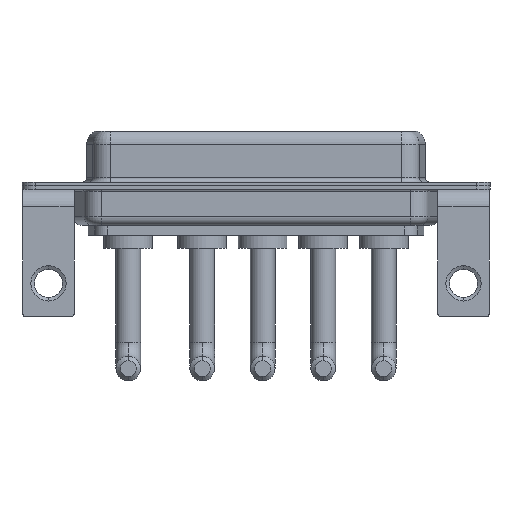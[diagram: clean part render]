
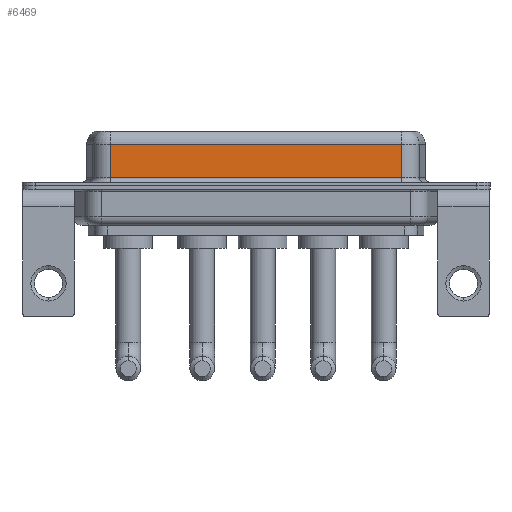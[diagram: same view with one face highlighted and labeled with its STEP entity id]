
A CAD part, front view. The second image highlights one B-rep face of the part: STEP entity #6469.
In plain terms, the highlighted planar face has unit normal (0, -1, 0).
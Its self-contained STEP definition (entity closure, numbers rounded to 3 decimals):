
#188 = CARTESIAN_POINT ( 'NONE',  ( 40.037, -3.95, 0.9 ) ) ;
#1151 = VERTEX_POINT ( 'NONE', #8753 ) ;
#1184 = VERTEX_POINT ( 'NONE', #9587 ) ;
#1342 = DIRECTION ( 'NONE',  ( 1., 0., 0. ) ) ;
#1754 = VECTOR ( 'NONE', #6107, 1000. ) ;
#1805 = VECTOR ( 'NONE', #10194, 1000. ) ;
#2110 = ORIENTED_EDGE ( 'NONE', *, *, #11694, .F. ) ;
#2788 = DIRECTION ( 'NONE',  ( 0., 0., 1. ) ) ;
#2907 = LINE ( 'NONE', #11428, #1754 ) ;
#2915 = LINE ( 'NONE', #6045, #1805 ) ;
#5626 = LINE ( 'NONE', #188, #5764 ) ;
#5632 = VERTEX_POINT ( 'NONE', #7070 ) ;
#5764 = VECTOR ( 'NONE', #1342, 1000. ) ;
#5887 = ORIENTED_EDGE ( 'NONE', *, *, #8038, .T. ) ;
#5916 = FACE_OUTER_BOUND ( 'NONE', #6732, .T. ) ;
#6045 = CARTESIAN_POINT ( 'NONE',  ( 40.037, -3.95, 4.65 ) ) ;
#6107 = DIRECTION ( 'NONE',  ( 0., 0., -1. ) ) ;
#6469 = ADVANCED_FACE ( 'NONE', ( #5916 ), #13076, .F. ) ;
#6732 = EDGE_LOOP ( 'NONE', ( #2110, #5887, #8091, #12828 ) ) ;
#7070 = CARTESIAN_POINT ( 'NONE',  ( 40.037, -3.95, 4.65 ) ) ;
#7898 = CARTESIAN_POINT ( 'NONE',  ( 40.037, -3.95, 6.4 ) ) ;
#8038 = EDGE_CURVE ( 'NONE', #5632, #12316, #2915, .T. ) ;
#8091 = ORIENTED_EDGE ( 'NONE', *, *, #11232, .T. ) ;
#8160 = CARTESIAN_POINT ( 'NONE',  ( 7.013, -3.95, 6.4 ) ) ;
#8227 = DIRECTION ( 'NONE',  ( 0., 0., -1. ) ) ;
#8753 = CARTESIAN_POINT ( 'NONE',  ( 40.037, -3.95, 0.9 ) ) ;
#9587 = CARTESIAN_POINT ( 'NONE',  ( 7.013, -3.95, 0.9 ) ) ;
#9903 = VECTOR ( 'NONE', #8227, 1000. ) ;
#10096 = AXIS2_PLACEMENT_3D ( 'NONE', #7898, #12054, #2788 ) ;
#10194 = DIRECTION ( 'NONE',  ( -1., 0., 0. ) ) ;
#11232 = EDGE_CURVE ( 'NONE', #12316, #1184, #12457, .T. ) ;
#11319 = EDGE_CURVE ( 'NONE', #1184, #1151, #5626, .T. ) ;
#11428 = CARTESIAN_POINT ( 'NONE',  ( 40.037, -3.95, 6.4 ) ) ;
#11694 = EDGE_CURVE ( 'NONE', #5632, #1151, #2907, .T. ) ;
#12054 = DIRECTION ( 'NONE',  ( 0., 1., 0. ) ) ;
#12316 = VERTEX_POINT ( 'NONE', #12627 ) ;
#12457 = LINE ( 'NONE', #8160, #9903 ) ;
#12627 = CARTESIAN_POINT ( 'NONE',  ( 7.013, -3.95, 4.65 ) ) ;
#12828 = ORIENTED_EDGE ( 'NONE', *, *, #11319, .T. ) ;
#13076 = PLANE ( 'NONE',  #10096 ) ;
